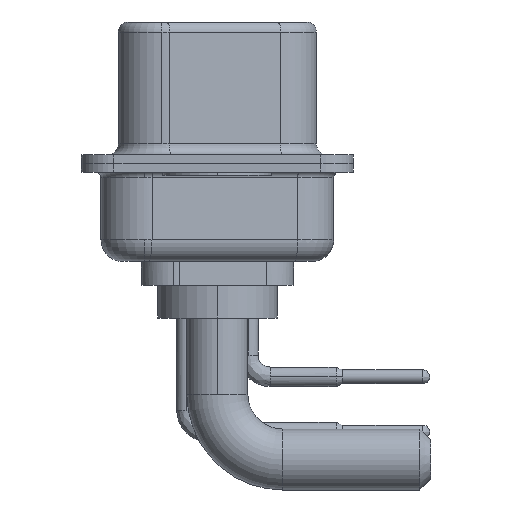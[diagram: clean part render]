
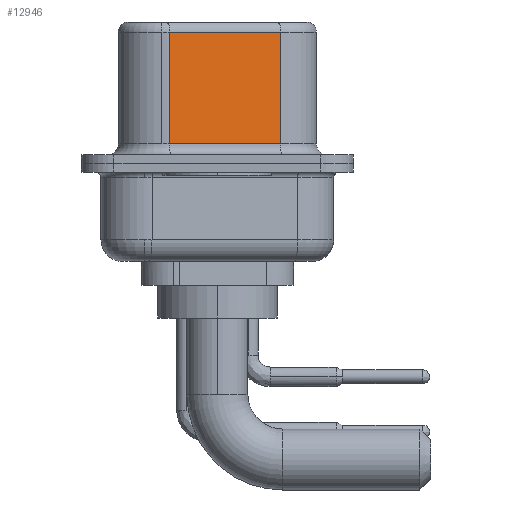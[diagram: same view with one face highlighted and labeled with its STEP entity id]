
A CAD part, left-side view. The second image highlights one B-rep face of the part: STEP entity #12946.
In plain terms, the highlighted planar face has unit normal (-0.985, -0.174, 0).
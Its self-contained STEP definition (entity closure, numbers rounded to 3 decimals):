
#589 = AXIS2_PLACEMENT_3D ( 'NONE', #3317, #5067, #6837 ) ;
#2291 = ORIENTED_EDGE ( 'NONE', *, *, #10966, .F. ) ;
#2447 = CARTESIAN_POINT ( 'NONE',  ( 3.68, 2.203, 0.9 ) ) ;
#3252 = CARTESIAN_POINT ( 'NONE',  ( 3.68, 2.203, 6.52 ) ) ;
#3317 = CARTESIAN_POINT ( 'NONE',  ( 4.58, -2.897, 6.52 ) ) ;
#3421 = FACE_OUTER_BOUND ( 'NONE', #8471, .T. ) ;
#4184 = DIRECTION ( 'NONE',  ( 0., 0., -1. ) ) ;
#4524 = DIRECTION ( 'NONE',  ( 0.174, -0.985, 0. ) ) ;
#4683 = ORIENTED_EDGE ( 'NONE', *, *, #10894, .T. ) ;
#4983 = VERTEX_POINT ( 'NONE', #16494 ) ;
#5067 = DIRECTION ( 'NONE',  ( 0.985, 0.174, 0. ) ) ;
#5307 = VERTEX_POINT ( 'NONE', #19435 ) ;
#5479 = VECTOR ( 'NONE', #12440, 1000. ) ;
#6837 = DIRECTION ( 'NONE',  ( -0.174, 0.985, 0. ) ) ;
#7335 = CARTESIAN_POINT ( 'NONE',  ( 4.58, -2.897, 0.9 ) ) ;
#8325 = VECTOR ( 'NONE', #4524, 1000. ) ;
#8471 = EDGE_LOOP ( 'NONE', ( #2291, #4683, #10736, #15445 ) ) ;
#9087 = LINE ( 'NONE', #15430, #13563 ) ;
#9413 = CARTESIAN_POINT ( 'NONE',  ( 4.58, -2.897, 6.02 ) ) ;
#9431 = EDGE_CURVE ( 'NONE', #4983, #20611, #17341, .T. ) ;
#10736 = ORIENTED_EDGE ( 'NONE', *, *, #9431, .T. ) ;
#10894 = EDGE_CURVE ( 'NONE', #13454, #4983, #16201, .T. ) ;
#10966 = EDGE_CURVE ( 'NONE', #13454, #5307, #9087, .T. ) ;
#12440 = DIRECTION ( 'NONE',  ( 0., 0., -1. ) ) ;
#12877 = DIRECTION ( 'NONE',  ( -0.174, 0.985, 0. ) ) ;
#12946 = ADVANCED_FACE ( 'NONE', ( #3421 ), #16027, .F. ) ;
#13454 = VERTEX_POINT ( 'NONE', #9413 ) ;
#13563 = VECTOR ( 'NONE', #4184, 1000. ) ;
#15044 = EDGE_CURVE ( 'NONE', #20611, #5307, #17039, .T. ) ;
#15430 = CARTESIAN_POINT ( 'NONE',  ( 4.58, -2.897, 6.52 ) ) ;
#15445 = ORIENTED_EDGE ( 'NONE', *, *, #15044, .T. ) ;
#15782 = CARTESIAN_POINT ( 'NONE',  ( 4.58, -2.897, 6.02 ) ) ;
#16027 = PLANE ( 'NONE',  #589 ) ;
#16201 = LINE ( 'NONE', #15782, #20581 ) ;
#16494 = CARTESIAN_POINT ( 'NONE',  ( 3.68, 2.203, 6.02 ) ) ;
#17039 = LINE ( 'NONE', #7335, #8325 ) ;
#17341 = LINE ( 'NONE', #3252, #5479 ) ;
#19435 = CARTESIAN_POINT ( 'NONE',  ( 4.58, -2.897, 0.9 ) ) ;
#20581 = VECTOR ( 'NONE', #12877, 1000. ) ;
#20611 = VERTEX_POINT ( 'NONE', #2447 ) ;
